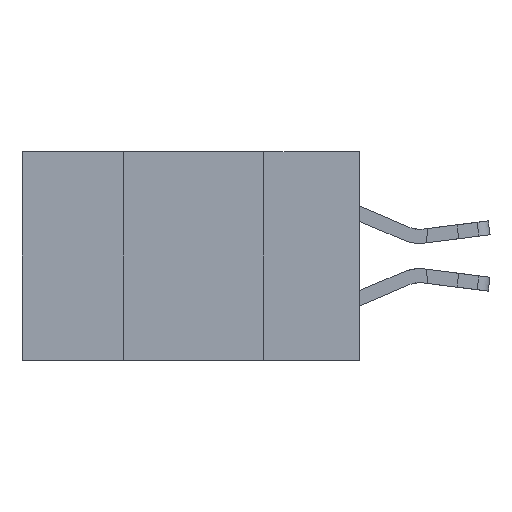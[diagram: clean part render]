
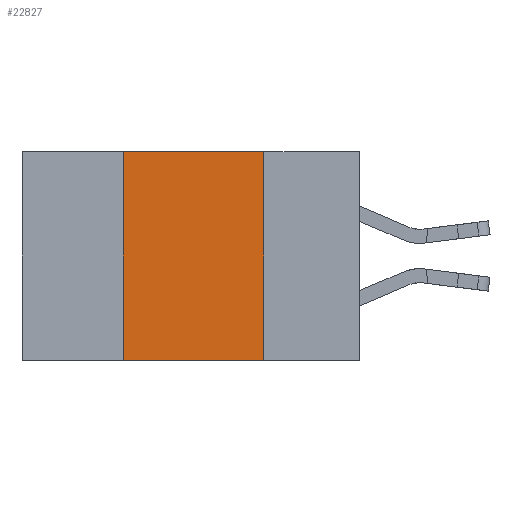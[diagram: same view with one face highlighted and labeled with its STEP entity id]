
A CAD part, left-side view. The second image highlights one B-rep face of the part: STEP entity #22827.
In plain terms, the highlighted planar face has unit normal (-1, 0, 0).
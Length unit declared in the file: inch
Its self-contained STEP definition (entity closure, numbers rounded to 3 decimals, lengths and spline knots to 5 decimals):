
#450 = DIRECTION ( 'NONE',  ( 0., -1., 0. ) ) ;
#2647 = VERTEX_POINT ( 'NONE', #4401 ) ;
#2769 = LINE ( 'NONE', #19317, #21662 ) ;
#2978 = AXIS2_PLACEMENT_3D ( 'NONE', #26466, #14942, #24187 ) ;
#3948 = ORIENTED_EDGE ( 'NONE', *, *, #4073, .T. ) ;
#4073 = EDGE_CURVE ( 'NONE', #22343, #8079, #16855, .T. ) ;
#4401 = CARTESIAN_POINT ( 'NONE',  ( 0., 0.42, 0. ) ) ;
#5953 = EDGE_CURVE ( 'NONE', #9499, #8079, #6708, .T. ) ;
#6708 = LINE ( 'NONE', #15954, #10675 ) ;
#7238 = CARTESIAN_POINT ( 'NONE',  ( 0., 0.17, -0.37 ) ) ;
#7985 = PLANE ( 'NONE',  #2978 ) ;
#8079 = VERTEX_POINT ( 'NONE', #7238 ) ;
#9499 = VERTEX_POINT ( 'NONE', #18620 ) ;
#10675 = VECTOR ( 'NONE', #25192, 39.37008 ) ;
#11089 = ORIENTED_EDGE ( 'NONE', *, *, #17592, .F. ) ;
#11966 = VECTOR ( 'NONE', #19612, 39.37008 ) ;
#14918 = EDGE_CURVE ( 'NONE', #22343, #2647, #2769, .T. ) ;
#14942 = DIRECTION ( 'NONE',  ( 1., 0., 0. ) ) ;
#15954 = CARTESIAN_POINT ( 'NONE',  ( 0., 0.17, 0. ) ) ;
#16855 = LINE ( 'NONE', #26096, #22711 ) ;
#17592 = EDGE_CURVE ( 'NONE', #2647, #9499, #17787, .T. ) ;
#17787 = LINE ( 'NONE', #22476, #11966 ) ;
#18620 = CARTESIAN_POINT ( 'NONE',  ( 0., 0.17, 0. ) ) ;
#19317 = CARTESIAN_POINT ( 'NONE',  ( 0., 0.42, 0. ) ) ;
#19612 = DIRECTION ( 'NONE',  ( 0., -1., 0. ) ) ;
#21662 = VECTOR ( 'NONE', #27944, 39.37008 ) ;
#22343 = VERTEX_POINT ( 'NONE', #28187 ) ;
#22476 = CARTESIAN_POINT ( 'NONE',  ( 0., 0.6, 0. ) ) ;
#22711 = VECTOR ( 'NONE', #450, 39.37008 ) ;
#22827 = ADVANCED_FACE ( 'NONE', ( #28738 ), #7985, .F. ) ;
#23603 = EDGE_LOOP ( 'NONE', ( #23604, #11089, #23609, #3948 ) ) ;
#23604 = ORIENTED_EDGE ( 'NONE', *, *, #5953, .F. ) ;
#23609 = ORIENTED_EDGE ( 'NONE', *, *, #14918, .F. ) ;
#24187 = DIRECTION ( 'NONE',  ( 0., 0., -1. ) ) ;
#25192 = DIRECTION ( 'NONE',  ( 0., 0., -1. ) ) ;
#26096 = CARTESIAN_POINT ( 'NONE',  ( 0., 0.6, -0.37 ) ) ;
#26466 = CARTESIAN_POINT ( 'NONE',  ( 0., 0.6, 0. ) ) ;
#27944 = DIRECTION ( 'NONE',  ( 0., 0., 1. ) ) ;
#28187 = CARTESIAN_POINT ( 'NONE',  ( 0., 0.42, -0.37 ) ) ;
#28738 = FACE_OUTER_BOUND ( 'NONE', #23603, .T. ) ;
